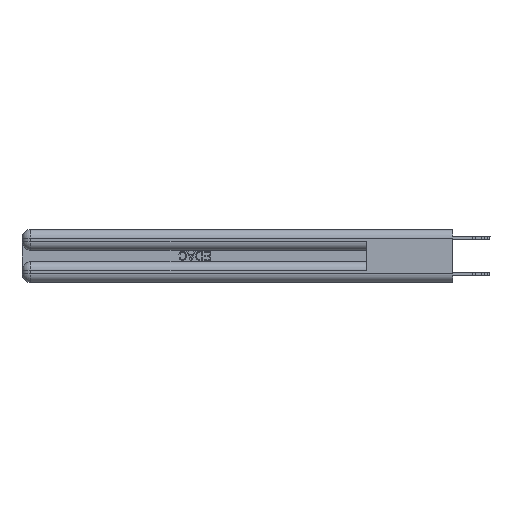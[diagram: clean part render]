
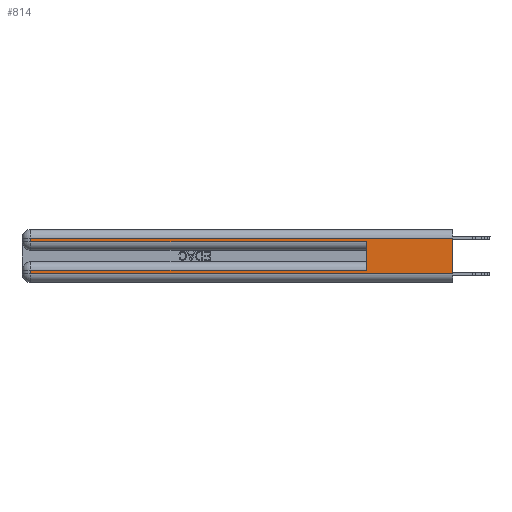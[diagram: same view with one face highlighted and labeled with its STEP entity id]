
A CAD part, left-side view. The second image highlights one B-rep face of the part: STEP entity #814.
In plain terms, the highlighted planar face has unit normal (-1, 0, 0).
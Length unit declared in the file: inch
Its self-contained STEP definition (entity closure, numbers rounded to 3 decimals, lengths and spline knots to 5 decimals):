
#86 = ORIENTED_EDGE ( 'NONE', *, *, #30587, .T. ) ;
#335 = LINE ( 'NONE', #28588, #30192 ) ;
#592 = CARTESIAN_POINT ( 'NONE',  ( 0., 2.94, 0.085 ) ) ;
#700 = VECTOR ( 'NONE', #14095, 39.37008 ) ;
#814 = ADVANCED_FACE ( 'NONE', ( #6376 ), #29492, .F. ) ;
#3521 = DIRECTION ( 'NONE',  ( 0., 0., -1. ) ) ;
#3848 = ORIENTED_EDGE ( 'NONE', *, *, #27880, .T. ) ;
#4313 = CARTESIAN_POINT ( 'NONE',  ( 0., 0.6, 0.285 ) ) ;
#4555 = CARTESIAN_POINT ( 'NONE',  ( 0., 0., 0.085 ) ) ;
#5814 = VECTOR ( 'NONE', #33537, 39.37008 ) ;
#5876 = CARTESIAN_POINT ( 'NONE',  ( 0., 0., 0.37 ) ) ;
#6376 = FACE_OUTER_BOUND ( 'NONE', #11106, .T. ) ;
#6771 = CARTESIAN_POINT ( 'NONE',  ( 0., 2.94, 0.37 ) ) ;
#6957 = VECTOR ( 'NONE', #3521, 39.37008 ) ;
#7170 = CARTESIAN_POINT ( 'NONE',  ( 0., 2.94, 0.37 ) ) ;
#7954 = AXIS2_PLACEMENT_3D ( 'NONE', #5876, #11361, #30178 ) ;
#9443 = CARTESIAN_POINT ( 'NONE',  ( 0., 0., 0.31 ) ) ;
#9785 = EDGE_CURVE ( 'NONE', #33091, #21014, #19934, .T. ) ;
#10428 = CARTESIAN_POINT ( 'NONE',  ( 0., 2.94, 0.06 ) ) ;
#10495 = VERTEX_POINT ( 'NONE', #592 ) ;
#10770 = VECTOR ( 'NONE', #20118, 39.37008 ) ;
#11106 = EDGE_LOOP ( 'NONE', ( #19418, #86, #13003, #3848, #30794, #22102, #13293, #18237 ) ) ;
#11291 = EDGE_CURVE ( 'NONE', #10495, #29872, #30244, .T. ) ;
#11361 = DIRECTION ( 'NONE',  ( 1., 0., 0. ) ) ;
#12130 = CARTESIAN_POINT ( 'NONE',  ( 0., 0., 0.37 ) ) ;
#13003 = ORIENTED_EDGE ( 'NONE', *, *, #9785, .T. ) ;
#13050 = DIRECTION ( 'NONE',  ( 0., -1., 0. ) ) ;
#13293 = ORIENTED_EDGE ( 'NONE', *, *, #11291, .T. ) ;
#13919 = LINE ( 'NONE', #24406, #700 ) ;
#14095 = DIRECTION ( 'NONE',  ( 0., -1., 0. ) ) ;
#14369 = DIRECTION ( 'NONE',  ( 0., 0., 1. ) ) ;
#15008 = DIRECTION ( 'NONE',  ( 0., 1., 0. ) ) ;
#15128 = CARTESIAN_POINT ( 'NONE',  ( 0., 2.94, 0.285 ) ) ;
#15464 = VERTEX_POINT ( 'NONE', #32299 ) ;
#18119 = CARTESIAN_POINT ( 'NONE',  ( 0., 0., 0.31 ) ) ;
#18237 = ORIENTED_EDGE ( 'NONE', *, *, #27564, .T. ) ;
#19418 = ORIENTED_EDGE ( 'NONE', *, *, #29783, .F. ) ;
#19595 = VERTEX_POINT ( 'NONE', #4313 ) ;
#19934 = LINE ( 'NONE', #7170, #5814 ) ;
#20118 = DIRECTION ( 'NONE',  ( 0., 1., 0. ) ) ;
#20461 = LINE ( 'NONE', #9443, #10770 ) ;
#21014 = VERTEX_POINT ( 'NONE', #15128 ) ;
#22102 = ORIENTED_EDGE ( 'NONE', *, *, #31541, .T. ) ;
#22624 = DIRECTION ( 'NONE',  ( 0., 0., -1. ) ) ;
#23372 = VECTOR ( 'NONE', #22624, 39.37008 ) ;
#24180 = CARTESIAN_POINT ( 'NONE',  ( 0., 2.94, 0.31 ) ) ;
#24406 = CARTESIAN_POINT ( 'NONE',  ( 0., 0., 0.06 ) ) ;
#27468 = CARTESIAN_POINT ( 'NONE',  ( 0., 0.6, 0.145 ) ) ;
#27564 = EDGE_CURVE ( 'NONE', #29872, #15464, #13919, .T. ) ;
#27880 = EDGE_CURVE ( 'NONE', #21014, #19595, #335, .T. ) ;
#27897 = CARTESIAN_POINT ( 'NONE',  ( 0., 0.6, 0.085 ) ) ;
#28120 = LINE ( 'NONE', #4555, #30104 ) ;
#28410 = VERTEX_POINT ( 'NONE', #18119 ) ;
#28588 = CARTESIAN_POINT ( 'NONE',  ( 0., 0., 0.285 ) ) ;
#28837 = VERTEX_POINT ( 'NONE', #27897 ) ;
#29492 = PLANE ( 'NONE',  #7954 ) ;
#29783 = EDGE_CURVE ( 'NONE', #28410, #15464, #30429, .T. ) ;
#29872 = VERTEX_POINT ( 'NONE', #10428 ) ;
#30094 = LINE ( 'NONE', #27468, #33907 ) ;
#30104 = VECTOR ( 'NONE', #15008, 39.37008 ) ;
#30178 = DIRECTION ( 'NONE',  ( 0., 0., -1. ) ) ;
#30192 = VECTOR ( 'NONE', #13050, 39.37008 ) ;
#30244 = LINE ( 'NONE', #6771, #6957 ) ;
#30429 = LINE ( 'NONE', #12130, #23372 ) ;
#30587 = EDGE_CURVE ( 'NONE', #28410, #33091, #20461, .T. ) ;
#30794 = ORIENTED_EDGE ( 'NONE', *, *, #31041, .F. ) ;
#31041 = EDGE_CURVE ( 'NONE', #28837, #19595, #30094, .T. ) ;
#31541 = EDGE_CURVE ( 'NONE', #28837, #10495, #28120, .T. ) ;
#32299 = CARTESIAN_POINT ( 'NONE',  ( 0., 0., 0.06 ) ) ;
#33091 = VERTEX_POINT ( 'NONE', #24180 ) ;
#33537 = DIRECTION ( 'NONE',  ( 0., 0., -1. ) ) ;
#33907 = VECTOR ( 'NONE', #14369, 39.37008 ) ;
